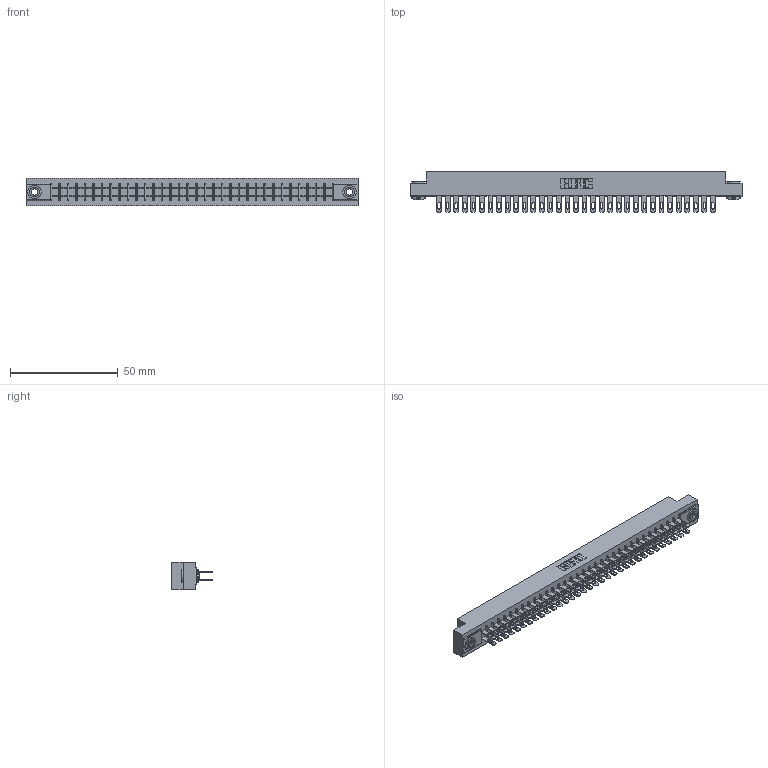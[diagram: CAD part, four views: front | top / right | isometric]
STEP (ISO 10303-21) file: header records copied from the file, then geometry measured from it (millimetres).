
FILE_DESCRIPTION (( 'STEP AP203' ), '1' );
FILE_NAME ('355-066-500-203.STEP', '2019-09-12T15:22:29', ( '' ), ( '' ), 'SwSTEP 2.0', 'SolidWorks 2016', '' );
FILE_SCHEMA (( 'CONFIG_CONTROL_DESIGN' ));
Length unit declared in the file: inch
Products named in the file (4): 345-250-002_345-250-002-102; 355-066-500-203; 305-290-001_500; 305 Part_.156 Dia
Assembly tree (69 placements, depth 2):
  355-066-500-203
    305 Part_.156 Dia
    305-290-001_500  x66
    345-250-002_345-250-002-102  x2
Bounding box: 153.77 x 18.85 x 12.7 mm (x, y, z)
Volume: 16188.3 mm3; surface area: 21941.3 mm2
Topology: 69 solids, 69 shells, 3468 faces, 9899 edges, 6418 vertices
Faces by surface type: plane 1940, cylinder 1388, sphere 132, cone 8
Entity records: 37913 total; most frequent: CARTESIAN_POINT 6254, ORIENTED_EDGE 6198, DIRECTION 6075, EDGE_CURVE 3099, LINE 2485, VECTOR 2485, VERTEX_POINT 1974, AXIS2_PLACEMENT_3D 1795
